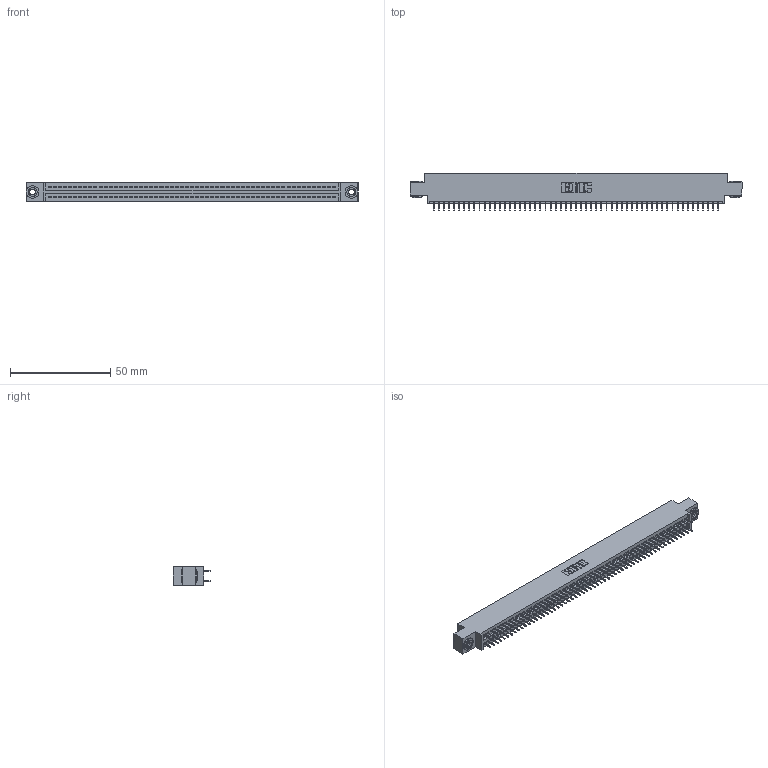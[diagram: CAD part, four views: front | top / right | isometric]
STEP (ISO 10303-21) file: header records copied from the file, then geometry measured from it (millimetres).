
FILE_DESCRIPTION (( 'STEP AP203' ), '1' );
FILE_NAME ('845-114-525-803.STEP', '2020-09-24T08:12:32', ( '' ), ( '' ), 'SwSTEP 2.0', 'SolidWorks 2020', '' );
FILE_SCHEMA (( 'CONFIG_CONTROL_DESIGN' ));
Length unit declared in the file: inch
Products named in the file (4): 845-114-525-803; 845 Part_0.170 Offset - 0.156 Dia-TH; 345-292-001_345-293-125; 345-250-002_345-250-002-102
Assembly tree (117 placements, depth 2):
  845-114-525-803
    845 Part_0.170 Offset - 0.156 Dia-TH
    345-292-001_345-293-125  x114
    345-250-002_345-250-002-102  x2
Bounding box: 165.99 x 18.72 x 9.4 mm (x, y, z)
Volume: 15981.9 mm3; surface area: 23697.4 mm2
Topology: 117 solids, 117 shells, 6324 faces, 17871 edges, 11454 vertices
Faces by surface type: plane 4540, cylinder 1776, cone 8
Entity records: 43560 total; most frequent: CARTESIAN_POINT 7263, ORIENTED_EDGE 7190, DIRECTION 6417, EDGE_CURVE 3595, LINE 3215, VECTOR 3215, VERTEX_POINT 2390, AXIS2_PLACEMENT_3D 1601
